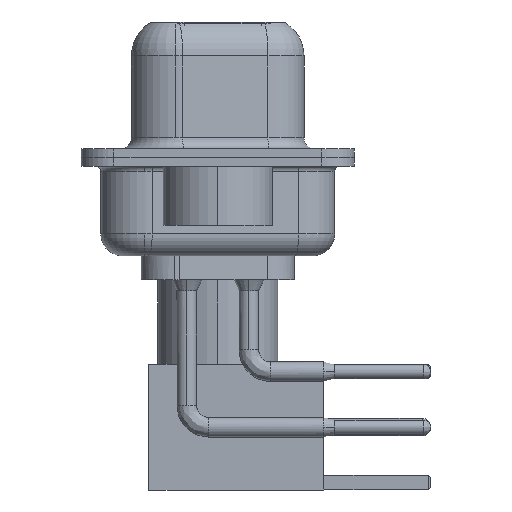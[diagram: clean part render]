
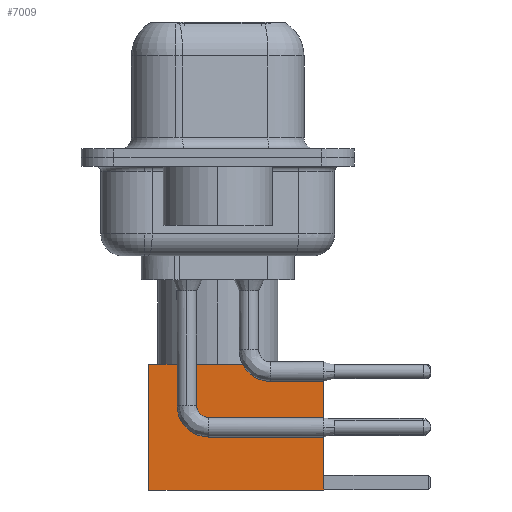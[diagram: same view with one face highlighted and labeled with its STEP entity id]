
A CAD part, left-side view. The second image highlights one B-rep face of the part: STEP entity #7009.
In plain terms, the highlighted face is planar.
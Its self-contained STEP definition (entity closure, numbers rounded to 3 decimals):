
#839 = EDGE_LOOP ( 'NONE', ( #10702, #2392, #13689, #15796 ) ) ;
#1704 = FACE_OUTER_BOUND ( 'NONE', #839, .T. ) ;
#1886 = VECTOR ( 'NONE', #16837, 1000. ) ;
#2003 = CARTESIAN_POINT ( 'NONE',  ( 0., 2.875, 8. ) ) ;
#2392 = ORIENTED_EDGE ( 'NONE', *, *, #5442, .T. ) ;
#2751 = VECTOR ( 'NONE', #12909, 1000. ) ;
#2914 = AXIS2_PLACEMENT_3D ( 'NONE', #3277, #14030, #12270 ) ;
#3277 = CARTESIAN_POINT ( 'NONE',  ( 2.875, 2.875, 0. ) ) ;
#4738 = PLANE ( 'NONE',  #2914 ) ;
#5442 = EDGE_CURVE ( 'NONE', #12841, #8235, #18402, .T. ) ;
#5783 = DIRECTION ( 'NONE',  ( 0., 0., -1. ) ) ;
#7009 = ADVANCED_FACE ( 'NONE', ( #1704 ), #4738, .T. ) ;
#8235 = VERTEX_POINT ( 'NONE', #8766 ) ;
#8586 = EDGE_CURVE ( 'NONE', #12397, #12841, #16225, .T. ) ;
#8766 = CARTESIAN_POINT ( 'NONE',  ( -2.875, 2.875, 0. ) ) ;
#10033 = DIRECTION ( 'NONE',  ( 0., 0., -1. ) ) ;
#10702 = ORIENTED_EDGE ( 'NONE', *, *, #8586, .T. ) ;
#10843 = CARTESIAN_POINT ( 'NONE',  ( 0., 2.875, 0. ) ) ;
#11343 = VECTOR ( 'NONE', #10033, 1000. ) ;
#11604 = CARTESIAN_POINT ( 'NONE',  ( -2.875, 2.875, 8. ) ) ;
#11932 = LINE ( 'NONE', #19205, #15527 ) ;
#12270 = DIRECTION ( 'NONE',  ( 0., 0., 1. ) ) ;
#12397 = VERTEX_POINT ( 'NONE', #14994 ) ;
#12841 = VERTEX_POINT ( 'NONE', #13118 ) ;
#12849 = EDGE_CURVE ( 'NONE', #17059, #8235, #11932, .T. ) ;
#12909 = DIRECTION ( 'NONE',  ( -1., 0., 0. ) ) ;
#13118 = CARTESIAN_POINT ( 'NONE',  ( 2.875, 2.875, 0. ) ) ;
#13268 = CARTESIAN_POINT ( 'NONE',  ( 2.875, 2.875, 0. ) ) ;
#13689 = ORIENTED_EDGE ( 'NONE', *, *, #12849, .F. ) ;
#14030 = DIRECTION ( 'NONE',  ( 0., 1., 0. ) ) ;
#14994 = CARTESIAN_POINT ( 'NONE',  ( 2.875, 2.875, 8. ) ) ;
#15527 = VECTOR ( 'NONE', #5783, 1000. ) ;
#15796 = ORIENTED_EDGE ( 'NONE', *, *, #19323, .F. ) ;
#16225 = LINE ( 'NONE', #13268, #11343 ) ;
#16837 = DIRECTION ( 'NONE',  ( -1., 0., 0. ) ) ;
#17059 = VERTEX_POINT ( 'NONE', #11604 ) ;
#18402 = LINE ( 'NONE', #10843, #1886 ) ;
#18541 = LINE ( 'NONE', #2003, #2751 ) ;
#19205 = CARTESIAN_POINT ( 'NONE',  ( -2.875, 2.875, 0. ) ) ;
#19323 = EDGE_CURVE ( 'NONE', #12397, #17059, #18541, .T. ) ;
